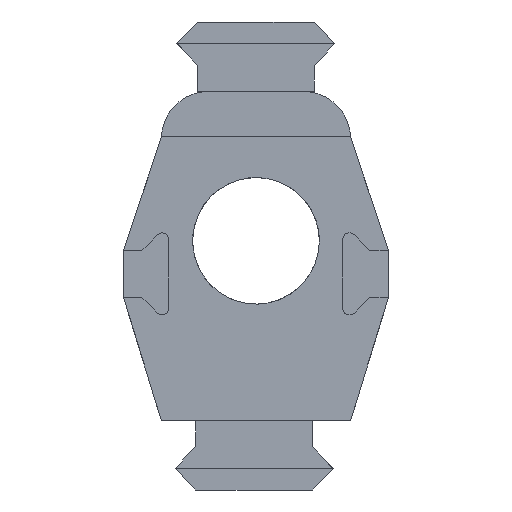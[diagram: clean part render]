
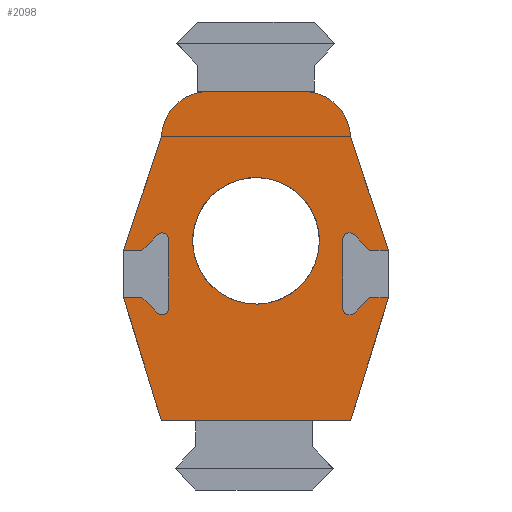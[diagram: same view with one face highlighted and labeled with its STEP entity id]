
A CAD part, front view. The second image highlights one B-rep face of the part: STEP entity #2098.
In plain terms, the highlighted planar face has unit normal (0, -1, 0).
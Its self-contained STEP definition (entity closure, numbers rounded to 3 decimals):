
#26=FACE_BOUND('',#225,.T.);
#31=ELLIPSE('',#2235,3.676,2.54);
#33=ELLIPSE('',#2237,3.676,2.54);
#52=CIRCLE('',#2224,0.889);
#54=CIRCLE('',#2228,0.889);
#56=CIRCLE('',#2239,0.889);
#57=CIRCLE('',#2240,0.889);
#58=CIRCLE('',#2241,6.35);
#59=CIRCLE('',#2242,6.35);
#60=CIRCLE('',#2243,8.5);
#61=CIRCLE('',#2244,8.5);
#107=FACE_OUTER_BOUND('',#224,.T.);
#224=EDGE_LOOP('',(#1419,#1420,#1421,#1422,#1423,#1424,#1425,#1426,#1427,
#1428,#1429,#1430,#1431,#1432,#1433,#1434,#1435,#1436,#1437,#1438,#1439,
#1440,#1441,#1442));
#225=EDGE_LOOP('',(#1443,#1444));
#335=LINE('',#2972,#599);
#340=LINE('',#2986,#604);
#344=LINE('',#2998,#608);
#347=LINE('',#3004,#611);
#350=LINE('',#3010,#614);
#359=LINE('',#3048,#623);
#360=LINE('',#3050,#624);
#361=LINE('',#3052,#625);
#362=LINE('',#3056,#626);
#363=LINE('',#3060,#627);
#364=LINE('',#3062,#628);
#365=LINE('',#3064,#629);
#366=LINE('',#3068,#630);
#367=LINE('',#3071,#631);
#368=LINE('',#3072,#632);
#369=LINE('',#3073,#633);
#599=VECTOR('',#2386,10.);
#604=VECTOR('',#2399,10.);
#608=VECTOR('',#2411,10.);
#611=VECTOR('',#2416,10.);
#614=VECTOR('',#2421,10.);
#623=VECTOR('',#2442,10.);
#624=VECTOR('',#2443,10.);
#625=VECTOR('',#2444,10.);
#626=VECTOR('',#2447,10.);
#627=VECTOR('',#2450,10.);
#628=VECTOR('',#2451,10.);
#629=VECTOR('',#2452,10.);
#630=VECTOR('',#2455,10.);
#631=VECTOR('',#2458,10.);
#632=VECTOR('',#2459,10.);
#633=VECTOR('',#2460,10.);
#863=VERTEX_POINT('',#2970);
#864=VERTEX_POINT('',#2971);
#867=VERTEX_POINT('',#2979);
#869=VERTEX_POINT('',#2985);
#871=VERTEX_POINT('',#2991);
#873=VERTEX_POINT('',#2997);
#875=VERTEX_POINT('',#3003);
#877=VERTEX_POINT('',#3009);
#882=VERTEX_POINT('',#3027);
#883=VERTEX_POINT('',#3029);
#886=VERTEX_POINT('',#3041);
#887=VERTEX_POINT('',#3043);
#888=VERTEX_POINT('',#3047);
#889=VERTEX_POINT('',#3049);
#890=VERTEX_POINT('',#3051);
#891=VERTEX_POINT('',#3053);
#892=VERTEX_POINT('',#3055);
#893=VERTEX_POINT('',#3057);
#894=VERTEX_POINT('',#3059);
#895=VERTEX_POINT('',#3061);
#896=VERTEX_POINT('',#3063);
#897=VERTEX_POINT('',#3065);
#898=VERTEX_POINT('',#3067);
#899=VERTEX_POINT('',#3069);
#900=VERTEX_POINT('',#3074);
#901=VERTEX_POINT('',#3075);
#1063=EDGE_CURVE('',#863,#864,#335,.T.);
#1067=EDGE_CURVE('',#867,#863,#52,.T.);
#1070=EDGE_CURVE('',#869,#867,#340,.T.);
#1073=EDGE_CURVE('',#871,#869,#54,.T.);
#1076=EDGE_CURVE('',#873,#871,#344,.T.);
#1079=EDGE_CURVE('',#864,#875,#347,.T.);
#1082=EDGE_CURVE('',#877,#873,#350,.T.);
#1089=EDGE_CURVE('',#883,#882,#31,.T.);
#1093=EDGE_CURVE('',#887,#886,#33,.T.);
#1095=EDGE_CURVE('',#886,#888,#359,.T.);
#1096=EDGE_CURVE('',#889,#888,#360,.T.);
#1097=EDGE_CURVE('',#890,#889,#361,.T.);
#1098=EDGE_CURVE('',#891,#890,#56,.T.);
#1099=EDGE_CURVE('',#892,#891,#362,.T.);
#1100=EDGE_CURVE('',#893,#892,#57,.T.);
#1101=EDGE_CURVE('',#894,#893,#363,.T.);
#1102=EDGE_CURVE('',#895,#894,#364,.T.);
#1103=EDGE_CURVE('',#895,#896,#365,.T.);
#1104=EDGE_CURVE('',#896,#897,#58,.T.);
#1105=EDGE_CURVE('',#897,#898,#366,.T.);
#1106=EDGE_CURVE('',#898,#899,#59,.T.);
#1107=EDGE_CURVE('',#899,#877,#367,.T.);
#1108=EDGE_CURVE('',#875,#883,#368,.T.);
#1109=EDGE_CURVE('',#882,#887,#369,.T.);
#1110=EDGE_CURVE('',#900,#901,#60,.T.);
#1111=EDGE_CURVE('',#901,#900,#61,.T.);
#1419=ORIENTED_EDGE('',*,*,#1093,.T.);
#1420=ORIENTED_EDGE('',*,*,#1095,.T.);
#1421=ORIENTED_EDGE('',*,*,#1096,.F.);
#1422=ORIENTED_EDGE('',*,*,#1097,.F.);
#1423=ORIENTED_EDGE('',*,*,#1098,.F.);
#1424=ORIENTED_EDGE('',*,*,#1099,.F.);
#1425=ORIENTED_EDGE('',*,*,#1100,.F.);
#1426=ORIENTED_EDGE('',*,*,#1101,.F.);
#1427=ORIENTED_EDGE('',*,*,#1102,.F.);
#1428=ORIENTED_EDGE('',*,*,#1103,.T.);
#1429=ORIENTED_EDGE('',*,*,#1104,.T.);
#1430=ORIENTED_EDGE('',*,*,#1105,.T.);
#1431=ORIENTED_EDGE('',*,*,#1106,.T.);
#1432=ORIENTED_EDGE('',*,*,#1107,.T.);
#1433=ORIENTED_EDGE('',*,*,#1082,.T.);
#1434=ORIENTED_EDGE('',*,*,#1076,.T.);
#1435=ORIENTED_EDGE('',*,*,#1073,.T.);
#1436=ORIENTED_EDGE('',*,*,#1070,.T.);
#1437=ORIENTED_EDGE('',*,*,#1067,.T.);
#1438=ORIENTED_EDGE('',*,*,#1063,.T.);
#1439=ORIENTED_EDGE('',*,*,#1079,.T.);
#1440=ORIENTED_EDGE('',*,*,#1108,.T.);
#1441=ORIENTED_EDGE('',*,*,#1089,.T.);
#1442=ORIENTED_EDGE('',*,*,#1109,.T.);
#1443=ORIENTED_EDGE('',*,*,#1110,.T.);
#1444=ORIENTED_EDGE('',*,*,#1111,.T.);
#2002=PLANE('',#2238);
#2098=ADVANCED_FACE('',(#107,#26),#2002,.F.);
#2224=AXIS2_PLACEMENT_3D('',#2980,#2392,#2393);
#2228=AXIS2_PLACEMENT_3D('',#2992,#2404,#2405);
#2235=AXIS2_PLACEMENT_3D('',#3030,#2431,#2432);
#2237=AXIS2_PLACEMENT_3D('',#3044,#2437,#2438);
#2238=AXIS2_PLACEMENT_3D('',#3046,#2440,#2441);
#2239=AXIS2_PLACEMENT_3D('',#3054,#2445,#2446);
#2240=AXIS2_PLACEMENT_3D('',#3058,#2448,#2449);
#2241=AXIS2_PLACEMENT_3D('',#3066,#2453,#2454);
#2242=AXIS2_PLACEMENT_3D('',#3070,#2456,#2457);
#2243=AXIS2_PLACEMENT_3D('',#3076,#2461,#2462);
#2244=AXIS2_PLACEMENT_3D('',#3077,#2463,#2464);
#2386=DIRECTION('',(-0.707,0.,0.707));
#2392=DIRECTION('center_axis',(0.,1.,0.));
#2393=DIRECTION('ref_axis',(1.,0.,0.));
#2399=DIRECTION('',(0.,0.,-1.));
#2404=DIRECTION('center_axis',(0.,1.,0.));
#2405=DIRECTION('ref_axis',(-0.707,0.,0.707));
#2411=DIRECTION('',(0.707,0.,0.707));
#2416=DIRECTION('',(-1.,0.,0.));
#2421=DIRECTION('',(1.,0.,0.001));
#2431=DIRECTION('center_axis',(0.,-1.,0.));
#2432=DIRECTION('ref_axis',(0.294,0.,-0.956));
#2437=DIRECTION('center_axis',(0.,-1.,0.));
#2438=DIRECTION('ref_axis',(-0.294,0.,-0.956));
#2440=DIRECTION('center_axis',(0.,1.,0.));
#2441=DIRECTION('ref_axis',(-1.,0.,0.));
#2442=DIRECTION('',(0.294,0.,0.956));
#2443=DIRECTION('',(1.,0.,0.));
#2444=DIRECTION('',(0.707,0.,0.707));
#2445=DIRECTION('center_axis',(0.,-1.,0.));
#2446=DIRECTION('ref_axis',(0.707,0.,-0.707));
#2447=DIRECTION('',(0.,0.,-1.));
#2448=DIRECTION('center_axis',(0.,-1.,0.));
#2449=DIRECTION('ref_axis',(-1.,0.,0.));
#2450=DIRECTION('',(-0.707,0.,0.707));
#2451=DIRECTION('',(-1.,0.,0.001));
#2452=DIRECTION('',(-0.316,0.,0.949));
#2453=DIRECTION('center_axis',(0.,-1.,0.));
#2454=DIRECTION('ref_axis',(0.999,0.,0.04));
#2455=DIRECTION('',(-1.,0.,0.));
#2456=DIRECTION('center_axis',(0.,-1.,0.));
#2457=DIRECTION('ref_axis',(-0.999,0.,0.04));
#2458=DIRECTION('',(-0.316,0.,-0.949));
#2459=DIRECTION('',(0.294,0.,-0.956));
#2460=DIRECTION('',(1.,0.,0.));
#2461=DIRECTION('center_axis',(0.,1.,0.));
#2462=DIRECTION('ref_axis',(-1.,0.,0.));
#2463=DIRECTION('center_axis',(0.,1.,0.));
#2464=DIRECTION('ref_axis',(-1.,0.,0.));
#2970=CARTESIAN_POINT('',(-13.243,171.04,1.736));
#2971=CARTESIAN_POINT('',(-15.317,171.04,3.81));
#2972=CARTESIAN_POINT('',(-11.086,171.04,-0.422));
#2979=CARTESIAN_POINT('',(-11.725,171.04,2.364));
#2980=CARTESIAN_POINT('Origin',(-12.614,171.04,2.364));
#2985=CARTESIAN_POINT('',(-11.725,171.04,11.609));
#2986=CARTESIAN_POINT('',(-11.725,171.04,8.979));
#2991=CARTESIAN_POINT('',(-13.243,171.04,12.238));
#2992=CARTESIAN_POINT('Origin',(-12.614,171.04,11.609));
#2997=CARTESIAN_POINT('',(-15.317,171.04,10.163));
#2998=CARTESIAN_POINT('',(-12.441,171.04,13.039));
#3003=CARTESIAN_POINT('',(-17.78,171.04,3.81));
#3004=CARTESIAN_POINT('',(-7.659,171.04,3.81));
#3009=CARTESIAN_POINT('',(-17.78,171.04,10.16));
#3010=CARTESIAN_POINT('',(-8.892,171.04,10.171));
#3027=CARTESIAN_POINT('',(-12.69,171.04,-12.699));
#3029=CARTESIAN_POINT('',(-12.794,171.04,-12.394));
#3030=CARTESIAN_POINT('Origin',(-10.366,171.04,-11.647));
#3041=CARTESIAN_POINT('',(12.794,171.04,-12.394));
#3043=CARTESIAN_POINT('',(12.69,171.04,-12.699));
#3044=CARTESIAN_POINT('Origin',(10.366,171.04,-11.647));
#3046=CARTESIAN_POINT('Origin',(0.,171.04,6.35));
#3047=CARTESIAN_POINT('',(17.78,171.04,3.81));
#3048=CARTESIAN_POINT('',(17.368,171.04,2.471));
#3049=CARTESIAN_POINT('',(15.24,171.04,3.81));
#3050=CARTESIAN_POINT('',(8.89,171.04,3.81));
#3051=CARTESIAN_POINT('',(13.166,171.04,1.736));
#3052=CARTESIAN_POINT('',(12.065,171.04,0.635));
#3053=CARTESIAN_POINT('',(11.648,171.04,2.364));
#3054=CARTESIAN_POINT('Origin',(12.537,171.04,2.364));
#3055=CARTESIAN_POINT('',(11.648,171.04,11.609));
#3056=CARTESIAN_POINT('',(11.648,171.04,4.357));
#3057=CARTESIAN_POINT('',(13.166,171.04,12.238));
#3058=CARTESIAN_POINT('Origin',(12.537,171.04,11.609));
#3059=CARTESIAN_POINT('',(15.24,171.04,10.163));
#3060=CARTESIAN_POINT('',(11.346,171.04,14.057));
#3061=CARTESIAN_POINT('',(17.78,171.04,10.16));
#3062=CARTESIAN_POINT('',(7.622,171.04,10.172));
#3063=CARTESIAN_POINT('',(12.7,171.04,25.4));
#3064=CARTESIAN_POINT('',(14.923,171.04,18.733));
#3065=CARTESIAN_POINT('',(6.355,171.04,31.496));
#3066=CARTESIAN_POINT('Origin',(6.355,171.04,25.146));
#3067=CARTESIAN_POINT('',(-6.355,171.04,31.496));
#3068=CARTESIAN_POINT('',(-6.35,171.04,31.496));
#3069=CARTESIAN_POINT('',(-12.7,171.04,25.4));
#3070=CARTESIAN_POINT('Origin',(-6.355,171.04,25.146));
#3071=CARTESIAN_POINT('',(-17.463,171.04,11.113));
#3072=CARTESIAN_POINT('',(-14.828,171.04,-5.784));
#3073=CARTESIAN_POINT('',(6.35,171.04,-12.699));
#3074=CARTESIAN_POINT('',(8.064,171.04,14.118));
#3075=CARTESIAN_POINT('',(8.5,171.04,11.43));
#3076=CARTESIAN_POINT('Origin',(0.,171.04,11.43));
#3077=CARTESIAN_POINT('Origin',(0.,171.04,11.43));
